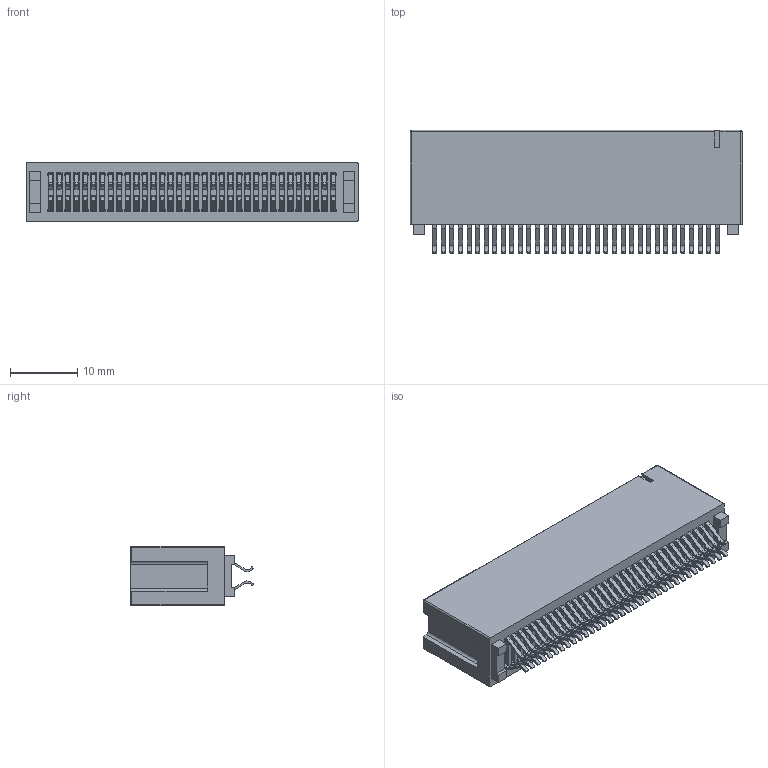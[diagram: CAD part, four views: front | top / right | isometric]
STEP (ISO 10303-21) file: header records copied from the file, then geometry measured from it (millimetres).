
FILE_DESCRIPTION (( 'STEP AP203' ), '1' );
FILE_NAME ('302-068-656-201.STEP', '2024-04-06T05:34:48', ( '' ), ( '' ), 'SwSTEP 2.0', 'SolidWorks 2023', '' );
FILE_SCHEMA (( 'CONFIG_CONTROL_DESIGN' ));
Length unit declared in the file: millimetre
Products named in the file (3): Contact_302-290-X56; HSG_Vertical HSG; 302-068-656-201
Assembly tree (69 placements, depth 2):
  302-068-656-201
    HSG_Vertical HSG
    Contact_302-290-X56  x68
Bounding box: 49.28 x 18.3 x 8.88 mm (x, y, z)
Volume: 3848 mm3; surface area: 10563.8 mm2
Topology: 69 solids, 69 shells, 3296 faces, 9824 edges, 6496 vertices
Faces by surface type: plane 2191, cylinder 1101, sphere 4
Entity records: 26955 total; most frequent: ORIENTED_EDGE 4632, CARTESIAN_POINT 4562, DIRECTION 3742, EDGE_CURVE 2316, LINE 2258, VECTOR 2258, VERTEX_POINT 1538, AXIS2_PLACEMENT_3D 742
